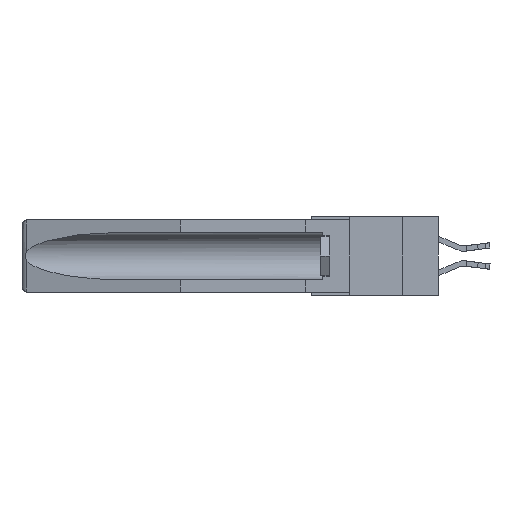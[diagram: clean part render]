
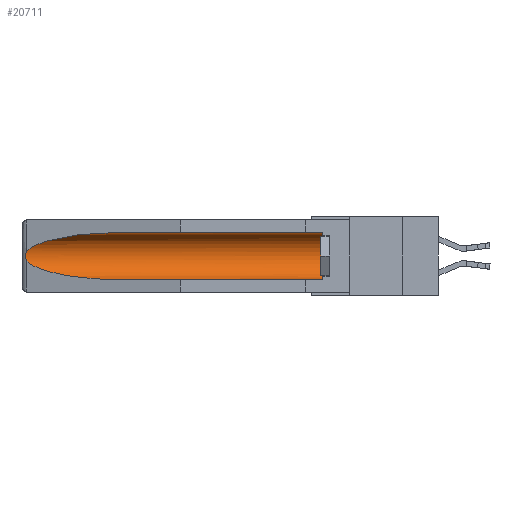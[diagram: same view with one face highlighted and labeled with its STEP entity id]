
A CAD part, left-side view. The second image highlights one B-rep face of the part: STEP entity #20711.
In plain terms, the highlighted cylindrical face has radius 2.857 mm (diameter 5.715 mm), a partial arc.
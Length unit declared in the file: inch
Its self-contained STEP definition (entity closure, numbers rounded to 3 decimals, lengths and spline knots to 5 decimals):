
#8 = CARTESIAN_POINT ( 'NONE',  ( 0.155, 0.126, -0.1715 ) ) ;
#55 = DIRECTION ( 'NONE',  ( 0., 1., 0. ) ) ;
#228 = DIRECTION ( 'NONE',  ( 0., 1., 0. ) ) ;
#799 = CARTESIAN_POINT ( 'NONE',  ( 0.155, 0.126, -0.284 ) ) ;
#919 = CARTESIAN_POINT ( 'NONE',  ( 0.26537, 1.52718, -0.19328 ) ) ;
#952 = VERTEX_POINT ( 'NONE', #27319 ) ;
#1351 = CARTESIAN_POINT ( 'NONE',  ( 0.2675, 1.53308, -0.16763 ) ) ;
#1353 = VERTEX_POINT ( 'NONE', #799 ) ;
#1623 = CARTESIAN_POINT ( 'NONE',  ( 0.26537, 1.52718, -0.19328 ) ) ;
#1634 = AXIS2_PLACEMENT_3D ( 'NONE', #8, #24187, #6346 ) ;
#1772 = DIRECTION ( 'NONE',  ( 0., 1., 0. ) ) ;
#2099 = ORIENTED_EDGE ( 'NONE', *, *, #21805, .T. ) ;
#2993 = CARTESIAN_POINT ( 'NONE',  ( 0.21114, 1.30732, -0.284 ) ) ;
#4017 = AXIS2_PLACEMENT_3D ( 'NONE', #24213, #228, #13161 ) ;
#4059 = ORIENTED_EDGE ( 'NONE', *, *, #8036, .F. ) ;
#4707 = VERTEX_POINT ( 'NONE', #919 ) ;
#6212 = CARTESIAN_POINT ( 'NONE',  ( 0.155, 0.126, -0.059 ) ) ;
#6346 = DIRECTION ( 'NONE',  ( 0., 0., 1. ) ) ;
#6637 = ORIENTED_EDGE ( 'NONE', *, *, #13717, .T. ) ;
#7048 = CARTESIAN_POINT ( 'NONE',  ( 0.25451, 1.48313, -0.09465 ) ) ;
#7051 = FACE_OUTER_BOUND ( 'NONE', #8317, .T. ) ;
#7897 = CARTESIAN_POINT ( 'NONE',  ( 0.26655, 1.53094, -0.18657 ) ) ;
#8036 = EDGE_CURVE ( 'NONE', #1353, #18652, #27907, .T. ) ;
#8317 = EDGE_LOOP ( 'NONE', ( #21495, #2099, #6637, #4059, #23274, #15066 ) ) ;
#9696 = VERTEX_POINT ( 'NONE', #14677 ) ;
#10472 = CARTESIAN_POINT ( 'NONE',  ( 0.2673, 1.5327, -0.16383 ) ) ;
#11717 = CIRCLE ( 'NONE', #1634, 0.1125 ) ;
#12552 = CARTESIAN_POINT ( 'NONE',  ( 0.26597, 1.5296, -0.19026 ) ) ;
#12639 = CARTESIAN_POINT ( 'NONE',  ( 0.2673, 1.53269, -0.17917 ) ) ;
#12975 = CARTESIAN_POINT ( 'NONE',  ( 0.155, 1.07973, -0.059 ) ) ;
#13161 = DIRECTION ( 'NONE',  ( 0., 0., 1. ) ) ;
#13178 = CARTESIAN_POINT ( 'NONE',  ( 0.155, -0.30754, -0.284 ) ) ;
#13717 = EDGE_CURVE ( 'NONE', #4707, #18652, #15747, .T. ) ;
#14677 = CARTESIAN_POINT ( 'NONE',  ( 0.155, 1.07973, -0.059 ) ) ;
#15066 = ORIENTED_EDGE ( 'NONE', *, *, #27006, .T. ) ;
#15196 = CARTESIAN_POINT ( 'NONE',  ( 0.21114, 1.30732, -0.059 ) ) ;
#15747 =( BOUNDED_CURVE ( )  B_SPLINE_CURVE ( 3, ( #20667, #25160, #2993, #18654 ),
 .UNSPECIFIED., .F., .T. ) 
 B_SPLINE_CURVE_WITH_KNOTS ( ( 4, 4 ),
 ( 0.1948, 1.5708 ),
 .UNSPECIFIED. ) 
 CURVE ( )  GEOMETRIC_REPRESENTATION_ITEM ( )  RATIONAL_B_SPLINE_CURVE ( ( 1., 0.848, 0.848, 1. ) ) 
 REPRESENTATION_ITEM ( '' )  );
#16710 = CARTESIAN_POINT ( 'NONE',  ( 0.26597, 1.52961, -0.15275 ) ) ;
#18265 = LINE ( 'NONE', #19724, #23066 ) ;
#18652 = VERTEX_POINT ( 'NONE', #27280 ) ;
#18654 = CARTESIAN_POINT ( 'NONE',  ( 0.155, 1.07973, -0.284 ) ) ;
#18857 = CARTESIAN_POINT ( 'NONE',  ( 0.26654, 1.53092, -0.15636 ) ) ;
#19724 = CARTESIAN_POINT ( 'NONE',  ( 0.155, -0.30754, -0.059 ) ) ;
#20318 =( BOUNDED_CURVE ( )  B_SPLINE_CURVE ( 3, ( #12975, #15196, #7048, #22025 ),
 .UNSPECIFIED., .F., .F. ) 
 B_SPLINE_CURVE_WITH_KNOTS ( ( 4, 4 ),
 ( 4.71239, 6.08839 ),
 .UNSPECIFIED. ) 
 CURVE ( )  GEOMETRIC_REPRESENTATION_ITEM ( )  RATIONAL_B_SPLINE_CURVE ( ( 1., 0.848, 0.848, 1. ) ) 
 REPRESENTATION_ITEM ( '' )  );
#20489 = VERTEX_POINT ( 'NONE', #6212 ) ;
#20667 = CARTESIAN_POINT ( 'NONE',  ( 0.26537, 1.52718, -0.19328 ) ) ;
#20711 = ADVANCED_FACE ( 'NONE', ( #7051 ), #27971, .F. ) ;
#20841 = B_SPLINE_CURVE_WITH_KNOTS ( 'NONE', 3,
 ( #23422, #16710, #18857, #10472, #1351, #25627, #12639, #7897, #12552, #1623 ),
 .UNSPECIFIED., .F., .F.,
 ( 4, 2, 2, 2, 4 ),
 ( 0., 0.00029, 0.00058, 0.00087, 0.00117 ),
 .UNSPECIFIED. ) ;
#21495 = ORIENTED_EDGE ( 'NONE', *, *, #22499, .T. ) ;
#21805 = EDGE_CURVE ( 'NONE', #952, #4707, #20841, .T. ) ;
#22025 = CARTESIAN_POINT ( 'NONE',  ( 0.26537, 1.52718, -0.14972 ) ) ;
#22499 = EDGE_CURVE ( 'NONE', #9696, #952, #20318, .T. ) ;
#22817 = EDGE_CURVE ( 'NONE', #1353, #20489, #11717, .T. ) ;
#23066 = VECTOR ( 'NONE', #1772, 39.37008 ) ;
#23274 = ORIENTED_EDGE ( 'NONE', *, *, #22817, .T. ) ;
#23422 = CARTESIAN_POINT ( 'NONE',  ( 0.26537, 1.52718, -0.14972 ) ) ;
#23456 = VECTOR ( 'NONE', #55, 39.37008 ) ;
#24187 = DIRECTION ( 'NONE',  ( 0., -1., 0. ) ) ;
#24213 = CARTESIAN_POINT ( 'NONE',  ( 0.155, -0.30754, -0.1715 ) ) ;
#25160 = CARTESIAN_POINT ( 'NONE',  ( 0.25451, 1.48313, -0.24835 ) ) ;
#25627 = CARTESIAN_POINT ( 'NONE',  ( 0.2675, 1.53308, -0.17534 ) ) ;
#27006 = EDGE_CURVE ( 'NONE', #20489, #9696, #18265, .T. ) ;
#27280 = CARTESIAN_POINT ( 'NONE',  ( 0.155, 1.07973, -0.284 ) ) ;
#27319 = CARTESIAN_POINT ( 'NONE',  ( 0.26537, 1.52718, -0.14972 ) ) ;
#27907 = LINE ( 'NONE', #13178, #23456 ) ;
#27971 = CYLINDRICAL_SURFACE ( 'NONE', #4017, 0.1125 ) ;
